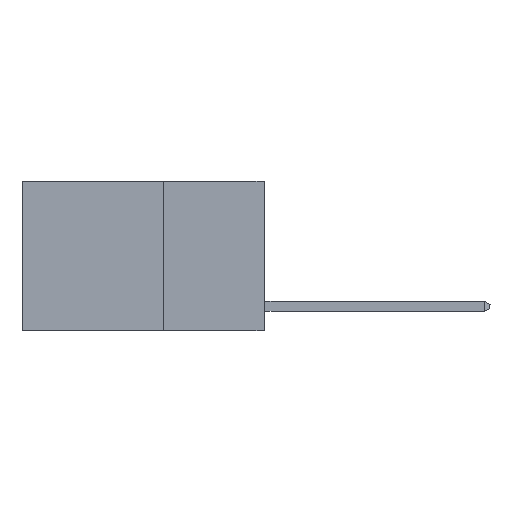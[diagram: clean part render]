
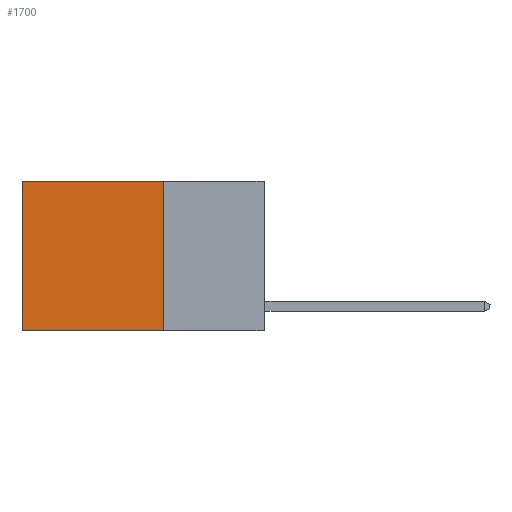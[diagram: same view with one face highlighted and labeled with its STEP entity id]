
A CAD part, left-side view. The second image highlights one B-rep face of the part: STEP entity #1700.
In plain terms, the highlighted planar face has unit normal (-1, 0, 0).
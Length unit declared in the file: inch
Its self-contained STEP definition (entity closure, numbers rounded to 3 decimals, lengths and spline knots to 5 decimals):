
#60 = AXIS2_PLACEMENT_3D ( 'NONE', #26378, #11965, #19783 ) ;
#809 = PLANE ( 'NONE',  #60 ) ;
#1700 = ADVANCED_FACE ( 'NONE', ( #19766 ), #809, .F. ) ;
#1802 = LINE ( 'NONE', #12316, #27110 ) ;
#5469 = VERTEX_POINT ( 'NONE', #11126 ) ;
#5873 = VECTOR ( 'NONE', #12488, 39.37008 ) ;
#6137 = VERTEX_POINT ( 'NONE', #26247 ) ;
#6971 = VERTEX_POINT ( 'NONE', #23728 ) ;
#7824 = EDGE_CURVE ( 'NONE', #21993, #5469, #9525, .T. ) ;
#8838 = DIRECTION ( 'NONE',  ( 0., 1., 0. ) ) ;
#8878 = EDGE_CURVE ( 'NONE', #6137, #6971, #1802, .T. ) ;
#9313 = EDGE_CURVE ( 'NONE', #21993, #6137, #18779, .T. ) ;
#9525 = LINE ( 'NONE', #12661, #5873 ) ;
#9724 = ORIENTED_EDGE ( 'NONE', *, *, #7824, .F. ) ;
#11060 = CARTESIAN_POINT ( 'NONE',  ( 0.2625, 0.25, 0. ) ) ;
#11126 = CARTESIAN_POINT ( 'NONE',  ( 0.2625, 0.25, -0.37 ) ) ;
#11232 = EDGE_LOOP ( 'NONE', ( #17990, #11537, #9724, #23352 ) ) ;
#11537 = ORIENTED_EDGE ( 'NONE', *, *, #16005, .F. ) ;
#11773 = VECTOR ( 'NONE', #8838, 39.37008 ) ;
#11965 = DIRECTION ( 'NONE',  ( 1., 0., 0. ) ) ;
#12316 = CARTESIAN_POINT ( 'NONE',  ( 0.2625, 0.6, 0. ) ) ;
#12488 = DIRECTION ( 'NONE',  ( 0., 0., -1. ) ) ;
#12661 = CARTESIAN_POINT ( 'NONE',  ( 0.2625, 0.25, 0. ) ) ;
#14858 = CARTESIAN_POINT ( 'NONE',  ( 0.2625, 0.25, 0. ) ) ;
#16005 = EDGE_CURVE ( 'NONE', #5469, #6971, #20902, .T. ) ;
#17009 = DIRECTION ( 'NONE',  ( 0., 0., -1. ) ) ;
#17990 = ORIENTED_EDGE ( 'NONE', *, *, #8878, .T. ) ;
#18588 = VECTOR ( 'NONE', #18948, 39.37008 ) ;
#18661 = CARTESIAN_POINT ( 'NONE',  ( 0.2625, 0.25, -0.37 ) ) ;
#18779 = LINE ( 'NONE', #11060, #11773 ) ;
#18948 = DIRECTION ( 'NONE',  ( 0., 1., 0. ) ) ;
#19766 = FACE_OUTER_BOUND ( 'NONE', #11232, .T. ) ;
#19783 = DIRECTION ( 'NONE',  ( 0., 0., -1. ) ) ;
#20902 = LINE ( 'NONE', #18661, #18588 ) ;
#21993 = VERTEX_POINT ( 'NONE', #14858 ) ;
#23352 = ORIENTED_EDGE ( 'NONE', *, *, #9313, .T. ) ;
#23728 = CARTESIAN_POINT ( 'NONE',  ( 0.2625, 0.6, -0.37 ) ) ;
#26247 = CARTESIAN_POINT ( 'NONE',  ( 0.2625, 0.6, 0. ) ) ;
#26378 = CARTESIAN_POINT ( 'NONE',  ( 0.2625, 0.25, 0. ) ) ;
#27110 = VECTOR ( 'NONE', #17009, 39.37008 ) ;
